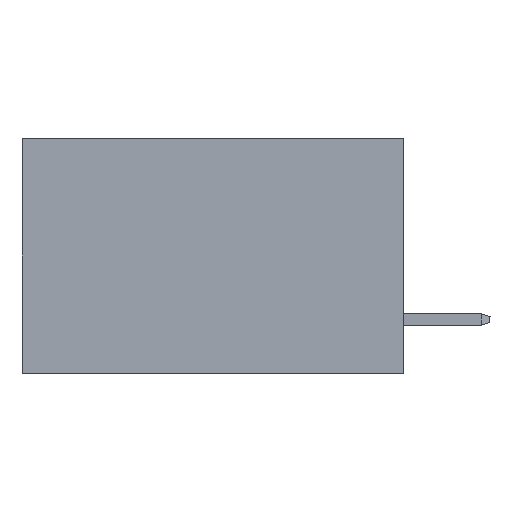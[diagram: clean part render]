
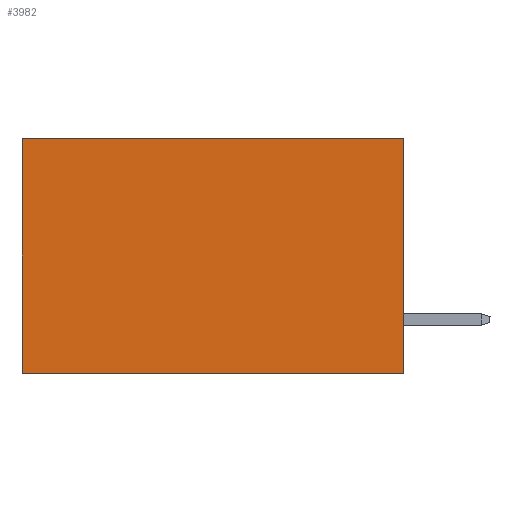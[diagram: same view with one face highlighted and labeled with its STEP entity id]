
A CAD part, left-side view. The second image highlights one B-rep face of the part: STEP entity #3982.
In plain terms, the highlighted planar face has unit normal (-1, 0, 0).
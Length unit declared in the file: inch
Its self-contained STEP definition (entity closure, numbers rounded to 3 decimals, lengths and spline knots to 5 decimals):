
#1004 = CARTESIAN_POINT ( 'NONE',  ( 0.2875, 0.6, 0. ) ) ;
#2837 = DIRECTION ( 'NONE',  ( 0., 1., 0. ) ) ;
#3982 = ADVANCED_FACE ( 'NONE', ( #13089 ), #8658, .F. ) ;
#4409 = DIRECTION ( 'NONE',  ( 0., 0., -1. ) ) ;
#5495 = VERTEX_POINT ( 'NONE', #13240 ) ;
#5694 = VECTOR ( 'NONE', #10591, 39.37008 ) ;
#6251 = ORIENTED_EDGE ( 'NONE', *, *, #11636, .T. ) ;
#7068 = ORIENTED_EDGE ( 'NONE', *, *, #17006, .T. ) ;
#7117 = DIRECTION ( 'NONE',  ( 0., 0., -1. ) ) ;
#8226 = ORIENTED_EDGE ( 'NONE', *, *, #22970, .F. ) ;
#8658 = PLANE ( 'NONE',  #10408 ) ;
#9669 = VECTOR ( 'NONE', #23359, 39.37008 ) ;
#9779 = ORIENTED_EDGE ( 'NONE', *, *, #21519, .F. ) ;
#10088 = EDGE_LOOP ( 'NONE', ( #7068, #8226, #9779, #6251 ) ) ;
#10408 = AXIS2_PLACEMENT_3D ( 'NONE', #14559, #22750, #4409 ) ;
#10591 = DIRECTION ( 'NONE',  ( 0., 1., 0. ) ) ;
#11636 = EDGE_CURVE ( 'NONE', #21242, #20629, #19158, .T. ) ;
#13089 = FACE_OUTER_BOUND ( 'NONE', #10088, .T. ) ;
#13107 = LINE ( 'NONE', #14981, #16735 ) ;
#13240 = CARTESIAN_POINT ( 'NONE',  ( 0.2875, 0., -0.37 ) ) ;
#13610 = VECTOR ( 'NONE', #7117, 39.37008 ) ;
#14559 = CARTESIAN_POINT ( 'NONE',  ( 0.2875, 0., 0. ) ) ;
#14981 = CARTESIAN_POINT ( 'NONE',  ( 0.2875, 0., -0.37 ) ) ;
#15145 = CARTESIAN_POINT ( 'NONE',  ( 0.2875, 0., 0. ) ) ;
#15539 = CARTESIAN_POINT ( 'NONE',  ( 0.2875, 0., 0. ) ) ;
#15964 = VERTEX_POINT ( 'NONE', #16473 ) ;
#16466 = CARTESIAN_POINT ( 'NONE',  ( 0.2875, 0.6, 0. ) ) ;
#16473 = CARTESIAN_POINT ( 'NONE',  ( 0.2875, 0.6, -0.37 ) ) ;
#16735 = VECTOR ( 'NONE', #2837, 39.37008 ) ;
#17006 = EDGE_CURVE ( 'NONE', #20629, #15964, #18913, .T. ) ;
#18913 = LINE ( 'NONE', #1004, #9669 ) ;
#19158 = LINE ( 'NONE', #15145, #5694 ) ;
#20629 = VERTEX_POINT ( 'NONE', #16466 ) ;
#21242 = VERTEX_POINT ( 'NONE', #22882 ) ;
#21519 = EDGE_CURVE ( 'NONE', #21242, #5495, #25485, .T. ) ;
#22750 = DIRECTION ( 'NONE',  ( 1., 0., 0. ) ) ;
#22882 = CARTESIAN_POINT ( 'NONE',  ( 0.2875, 0., 0. ) ) ;
#22970 = EDGE_CURVE ( 'NONE', #5495, #15964, #13107, .T. ) ;
#23359 = DIRECTION ( 'NONE',  ( 0., 0., -1. ) ) ;
#25485 = LINE ( 'NONE', #15539, #13610 ) ;
